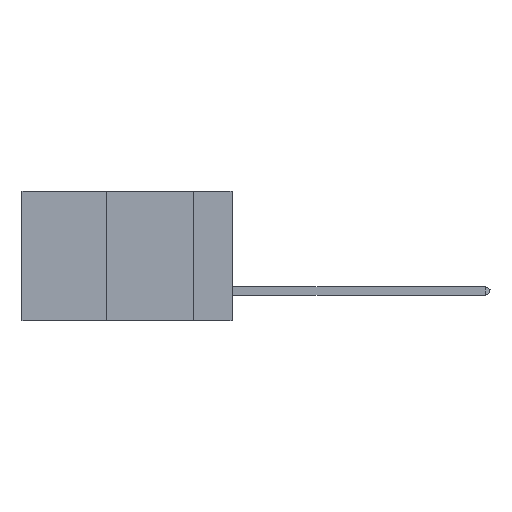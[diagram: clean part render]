
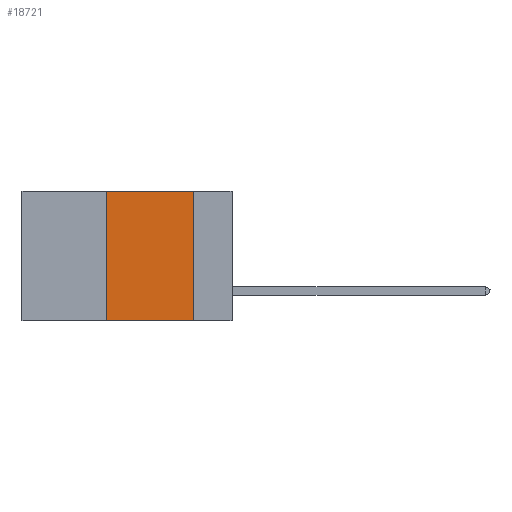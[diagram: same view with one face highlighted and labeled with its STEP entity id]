
A CAD part, left-side view. The second image highlights one B-rep face of the part: STEP entity #18721.
In plain terms, the highlighted planar face has unit normal (-1, 0, 0).
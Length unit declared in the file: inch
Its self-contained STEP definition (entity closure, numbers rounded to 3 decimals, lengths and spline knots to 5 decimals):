
#75 = LINE ( 'NONE', #12266, #10644 ) ;
#1182 = LINE ( 'NONE', #2010, #23554 ) ;
#1529 = VECTOR ( 'NONE', #6508, 39.37008 ) ;
#2010 = CARTESIAN_POINT ( 'NONE',  ( 0., 0.11, 0. ) ) ;
#3204 = LINE ( 'NONE', #13889, #1529 ) ;
#3269 = CARTESIAN_POINT ( 'NONE',  ( 0., 0.6, 0. ) ) ;
#3467 = VERTEX_POINT ( 'NONE', #22658 ) ;
#3771 = LINE ( 'NONE', #14229, #17359 ) ;
#3825 = ORIENTED_EDGE ( 'NONE', *, *, #5827, .F. ) ;
#5827 = EDGE_CURVE ( 'NONE', #3467, #11721, #3204, .T. ) ;
#6508 = DIRECTION ( 'NONE',  ( 0., -1., 0. ) ) ;
#7784 = EDGE_CURVE ( 'NONE', #11721, #18185, #1182, .T. ) ;
#7821 = EDGE_CURVE ( 'NONE', #20422, #3467, #75, .T. ) ;
#8561 = DIRECTION ( 'NONE',  ( 0., -1., 0. ) ) ;
#8738 = PLANE ( 'NONE',  #15289 ) ;
#9307 = EDGE_LOOP ( 'NONE', ( #15546, #3825, #20438, #18744 ) ) ;
#9660 = DIRECTION ( 'NONE',  ( 0., 0., -1. ) ) ;
#10644 = VECTOR ( 'NONE', #15189, 39.37008 ) ;
#10947 = EDGE_CURVE ( 'NONE', #20422, #18185, #3771, .T. ) ;
#11721 = VERTEX_POINT ( 'NONE', #21454 ) ;
#12104 = CARTESIAN_POINT ( 'NONE',  ( 0., 0.11, -0.37 ) ) ;
#12266 = CARTESIAN_POINT ( 'NONE',  ( 0., 0.36, 0. ) ) ;
#13889 = CARTESIAN_POINT ( 'NONE',  ( 0., 0.6, 0. ) ) ;
#14229 = CARTESIAN_POINT ( 'NONE',  ( 0., 0.6, -0.37 ) ) ;
#15189 = DIRECTION ( 'NONE',  ( 0., 0., 1. ) ) ;
#15289 = AXIS2_PLACEMENT_3D ( 'NONE', #3269, #19897, #19730 ) ;
#15546 = ORIENTED_EDGE ( 'NONE', *, *, #7784, .F. ) ;
#15762 = CARTESIAN_POINT ( 'NONE',  ( 0., 0.36, -0.37 ) ) ;
#17359 = VECTOR ( 'NONE', #8561, 39.37008 ) ;
#17635 = FACE_OUTER_BOUND ( 'NONE', #9307, .T. ) ;
#18185 = VERTEX_POINT ( 'NONE', #12104 ) ;
#18721 = ADVANCED_FACE ( 'NONE', ( #17635 ), #8738, .F. ) ;
#18744 = ORIENTED_EDGE ( 'NONE', *, *, #10947, .T. ) ;
#19730 = DIRECTION ( 'NONE',  ( 0., 0., -1. ) ) ;
#19897 = DIRECTION ( 'NONE',  ( 1., 0., 0. ) ) ;
#20422 = VERTEX_POINT ( 'NONE', #15762 ) ;
#20438 = ORIENTED_EDGE ( 'NONE', *, *, #7821, .F. ) ;
#21454 = CARTESIAN_POINT ( 'NONE',  ( 0., 0.11, 0. ) ) ;
#22658 = CARTESIAN_POINT ( 'NONE',  ( 0., 0.36, 0. ) ) ;
#23554 = VECTOR ( 'NONE', #9660, 39.37008 ) ;
